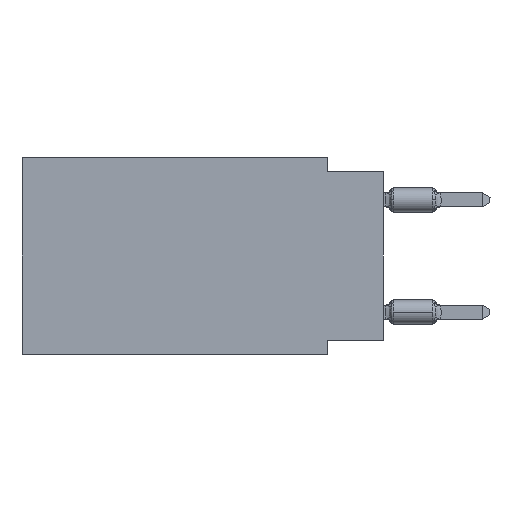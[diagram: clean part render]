
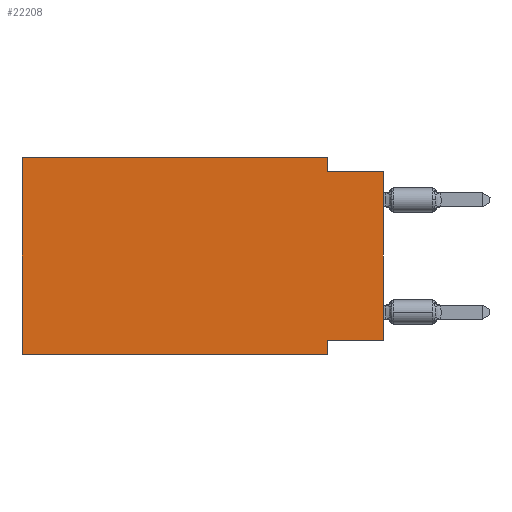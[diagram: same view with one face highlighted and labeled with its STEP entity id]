
A CAD part, left-side view. The second image highlights one B-rep face of the part: STEP entity #22208.
In plain terms, the highlighted planar face has unit normal (-1, 0, 0).
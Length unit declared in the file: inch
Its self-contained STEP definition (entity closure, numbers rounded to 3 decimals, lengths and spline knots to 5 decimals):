
#1084 = ORIENTED_EDGE ( 'NONE', *, *, #30889, .F. ) ;
#2536 = VERTEX_POINT ( 'NONE', #61363 ) ;
#5141 = LINE ( 'NONE', #5458, #9959 ) ;
#5458 = CARTESIAN_POINT ( 'NONE',  ( 0., 0.1, 0. ) ) ;
#5800 = DIRECTION ( 'NONE',  ( 0., 0., 1. ) ) ;
#7191 = VECTOR ( 'NONE', #53764, 39.37008 ) ;
#7373 = VECTOR ( 'NONE', #5800, 39.37008 ) ;
#7875 = LINE ( 'NONE', #18429, #12516 ) ;
#9575 = PLANE ( 'NONE',  #37807 ) ;
#9959 = VECTOR ( 'NONE', #56360, 39.37008 ) ;
#11067 = VECTOR ( 'NONE', #50834, 39.37008 ) ;
#12516 = VECTOR ( 'NONE', #41081, 39.37008 ) ;
#13126 = VERTEX_POINT ( 'NONE', #59658 ) ;
#14831 = DIRECTION ( 'NONE',  ( 1., 0., 0. ) ) ;
#16994 = DIRECTION ( 'NONE',  ( 0., -1., 0. ) ) ;
#17966 = ORIENTED_EDGE ( 'NONE', *, *, #52586, .T. ) ;
#18429 = CARTESIAN_POINT ( 'NONE',  ( 0., 0., -0.325 ) ) ;
#18515 = CARTESIAN_POINT ( 'NONE',  ( 0., 0., 0. ) ) ;
#19068 = VERTEX_POINT ( 'NONE', #26581 ) ;
#20091 = FACE_OUTER_BOUND ( 'NONE', #42950, .T. ) ;
#21873 = CARTESIAN_POINT ( 'NONE',  ( 0., 0., -0.025 ) ) ;
#22208 = ADVANCED_FACE ( 'NONE', ( #20091 ), #9575, .F. ) ;
#22581 = CARTESIAN_POINT ( 'NONE',  ( 0., 0.645, 0. ) ) ;
#22844 = DIRECTION ( 'NONE',  ( 0., 0., 1. ) ) ;
#24305 = ORIENTED_EDGE ( 'NONE', *, *, #35156, .F. ) ;
#26581 = CARTESIAN_POINT ( 'NONE',  ( 0., 0., -0.325 ) ) ;
#28901 = EDGE_CURVE ( 'NONE', #45079, #37563, #54087, .T. ) ;
#29411 = VECTOR ( 'NONE', #22844, 39.37008 ) ;
#29419 = CARTESIAN_POINT ( 'NONE',  ( 0., 0.645, 0. ) ) ;
#29486 = CARTESIAN_POINT ( 'NONE',  ( 0., 0.645, 0. ) ) ;
#30889 = EDGE_CURVE ( 'NONE', #57671, #32747, #39611, .T. ) ;
#31181 = ORIENTED_EDGE ( 'NONE', *, *, #28901, .F. ) ;
#31938 = ORIENTED_EDGE ( 'NONE', *, *, #49415, .T. ) ;
#32747 = VERTEX_POINT ( 'NONE', #29486 ) ;
#32963 = ORIENTED_EDGE ( 'NONE', *, *, #51730, .F. ) ;
#33143 = CARTESIAN_POINT ( 'NONE',  ( 0., 0.645, 0. ) ) ;
#33624 = CARTESIAN_POINT ( 'NONE',  ( 0., 0.645, -0.35 ) ) ;
#35156 = EDGE_CURVE ( 'NONE', #2536, #47119, #36574, .T. ) ;
#36574 = LINE ( 'NONE', #50540, #11067 ) ;
#37563 = VERTEX_POINT ( 'NONE', #21873 ) ;
#37807 = AXIS2_PLACEMENT_3D ( 'NONE', #33143, #14831, #47152 ) ;
#38021 = EDGE_CURVE ( 'NONE', #32747, #13126, #49320, .T. ) ;
#39606 = LINE ( 'NONE', #49265, #55038 ) ;
#39611 = LINE ( 'NONE', #29419, #7373 ) ;
#41081 = DIRECTION ( 'NONE',  ( 0., 1., 0. ) ) ;
#42688 = LINE ( 'NONE', #18515, #29411 ) ;
#42950 = EDGE_LOOP ( 'NONE', ( #17966, #31181, #59495, #44719, #1084, #31938, #24305, #32963 ) ) ;
#44719 = ORIENTED_EDGE ( 'NONE', *, *, #38021, .F. ) ;
#45079 = VERTEX_POINT ( 'NONE', #46698 ) ;
#46698 = CARTESIAN_POINT ( 'NONE',  ( 0., 0.1, -0.025 ) ) ;
#47119 = VERTEX_POINT ( 'NONE', #55825 ) ;
#47152 = DIRECTION ( 'NONE',  ( 0., 0., -1. ) ) ;
#49265 = CARTESIAN_POINT ( 'NONE',  ( 0., 0.645, -0.35 ) ) ;
#49320 = LINE ( 'NONE', #22581, #60714 ) ;
#49415 = EDGE_CURVE ( 'NONE', #57671, #47119, #39606, .T. ) ;
#50540 = CARTESIAN_POINT ( 'NONE',  ( 0., 0.1, -0.35 ) ) ;
#50834 = DIRECTION ( 'NONE',  ( 0., 0., -1. ) ) ;
#51730 = EDGE_CURVE ( 'NONE', #19068, #2536, #7875, .T. ) ;
#52586 = EDGE_CURVE ( 'NONE', #19068, #37563, #42688, .T. ) ;
#53764 = DIRECTION ( 'NONE',  ( 0., -1., 0. ) ) ;
#54087 = LINE ( 'NONE', #59626, #7191 ) ;
#55038 = VECTOR ( 'NONE', #59151, 39.37008 ) ;
#55825 = CARTESIAN_POINT ( 'NONE',  ( 0., 0.1, -0.35 ) ) ;
#56360 = DIRECTION ( 'NONE',  ( 0., 0., -1. ) ) ;
#57671 = VERTEX_POINT ( 'NONE', #33624 ) ;
#59151 = DIRECTION ( 'NONE',  ( 0., -1., 0. ) ) ;
#59415 = EDGE_CURVE ( 'NONE', #13126, #45079, #5141, .T. ) ;
#59495 = ORIENTED_EDGE ( 'NONE', *, *, #59415, .F. ) ;
#59626 = CARTESIAN_POINT ( 'NONE',  ( 0., 0., -0.025 ) ) ;
#59658 = CARTESIAN_POINT ( 'NONE',  ( 0., 0.1, 0. ) ) ;
#60714 = VECTOR ( 'NONE', #16994, 39.37008 ) ;
#61363 = CARTESIAN_POINT ( 'NONE',  ( 0., 0.1, -0.325 ) ) ;
